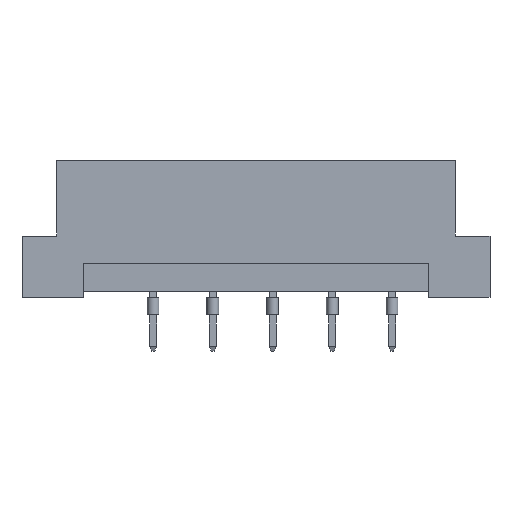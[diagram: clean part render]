
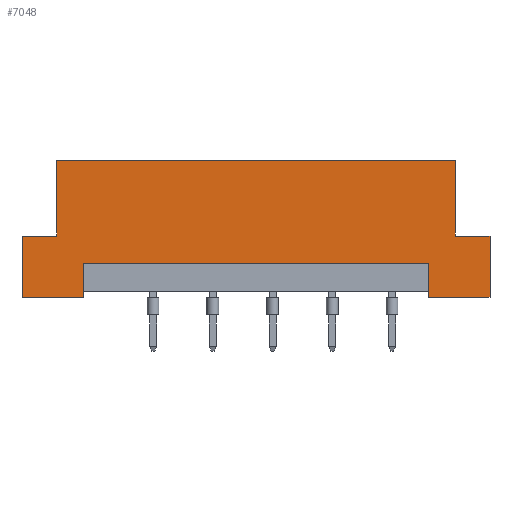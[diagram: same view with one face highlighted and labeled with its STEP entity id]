
A CAD part, front view. The second image highlights one B-rep face of the part: STEP entity #7048.
In plain terms, the highlighted planar face has unit normal (0, -1, 0).
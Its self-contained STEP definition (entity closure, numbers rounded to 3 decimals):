
#90 = DIRECTION ( 'NONE',  ( 0., 1., 0. ) ) ;
#134 = VERTEX_POINT ( 'NONE', #6791 ) ;
#160 = EDGE_CURVE ( 'NONE', #5860, #134, #2543, .T. ) ;
#199 = ORIENTED_EDGE ( 'NONE', *, *, #4637, .F. ) ;
#377 = VECTOR ( 'NONE', #6866, 1000. ) ;
#408 = LINE ( 'NONE', #2634, #3359 ) ;
#445 = ORIENTED_EDGE ( 'NONE', *, *, #2187, .F. ) ;
#552 = DIRECTION ( 'NONE',  ( -1., 0., 0. ) ) ;
#680 = VECTOR ( 'NONE', #4980, 1000. ) ;
#683 = ORIENTED_EDGE ( 'NONE', *, *, #3995, .F. ) ;
#708 = ORIENTED_EDGE ( 'NONE', *, *, #6460, .F. ) ;
#858 = VECTOR ( 'NONE', #6327, 1000. ) ;
#861 = VERTEX_POINT ( 'NONE', #6734 ) ;
#906 = CARTESIAN_POINT ( 'NONE',  ( 19.9, 0., 0. ) ) ;
#952 = LINE ( 'NONE', #2684, #6837 ) ;
#1167 = VERTEX_POINT ( 'NONE', #5324 ) ;
#1282 = LINE ( 'NONE', #3361, #4020 ) ;
#1418 = ORIENTED_EDGE ( 'NONE', *, *, #2986, .F. ) ;
#1699 = CARTESIAN_POINT ( 'NONE',  ( -16.94, 0., 11.6 ) ) ;
#1793 = ORIENTED_EDGE ( 'NONE', *, *, #6043, .F. ) ;
#2003 = LINE ( 'NONE', #2671, #4045 ) ;
#2011 = EDGE_LOOP ( 'NONE', ( #5216, #4098, #4525, #445, #6843, #6294, #1793, #5150, #199, #1418, #708, #683 ) ) ;
#2084 = DIRECTION ( 'NONE',  ( 0., 0., -1. ) ) ;
#2187 = EDGE_CURVE ( 'NONE', #4415, #5860, #4401, .T. ) ;
#2193 = LINE ( 'NONE', #3847, #4277 ) ;
#2227 = CARTESIAN_POINT ( 'NONE',  ( -16.94, 0., 5.2 ) ) ;
#2368 = CARTESIAN_POINT ( 'NONE',  ( -14.69, 0., 0.5 ) ) ;
#2543 = LINE ( 'NONE', #3081, #377 ) ;
#2559 = VERTEX_POINT ( 'NONE', #1699 ) ;
#2571 = DIRECTION ( 'NONE',  ( 1., 0., 0. ) ) ;
#2602 = DIRECTION ( 'NONE',  ( 1., 0., 0. ) ) ;
#2634 = CARTESIAN_POINT ( 'NONE',  ( -19.9, 0., 11.6 ) ) ;
#2671 = CARTESIAN_POINT ( 'NONE',  ( 19.9, 0., 5.2 ) ) ;
#2684 = CARTESIAN_POINT ( 'NONE',  ( 14.69, 0., 0.5 ) ) ;
#2693 = CARTESIAN_POINT ( 'NONE',  ( -19.9, 0., 5.2 ) ) ;
#2758 = VERTEX_POINT ( 'NONE', #2227 ) ;
#2821 = VECTOR ( 'NONE', #6826, 1000. ) ;
#2983 = CARTESIAN_POINT ( 'NONE',  ( 16.94, 0., 5.2 ) ) ;
#2986 = EDGE_CURVE ( 'NONE', #4608, #861, #1282, .T. ) ;
#3016 = LINE ( 'NONE', #6293, #858 ) ;
#3081 = CARTESIAN_POINT ( 'NONE',  ( -19.9, 0., 0. ) ) ;
#3222 = CARTESIAN_POINT ( 'NONE',  ( 14.69, 0., 2.9 ) ) ;
#3250 = CARTESIAN_POINT ( 'NONE',  ( -14.69, 0., 2.9 ) ) ;
#3359 = VECTOR ( 'NONE', #2571, 1000. ) ;
#3361 = CARTESIAN_POINT ( 'NONE',  ( -19.9, 0., 0. ) ) ;
#3554 = VERTEX_POINT ( 'NONE', #2983 ) ;
#3674 = VERTEX_POINT ( 'NONE', #5849 ) ;
#3776 = EDGE_CURVE ( 'NONE', #5462, #134, #952, .T. ) ;
#3824 = VECTOR ( 'NONE', #7015, 1000. ) ;
#3847 = CARTESIAN_POINT ( 'NONE',  ( -19.9, 0., 0. ) ) ;
#3926 = VECTOR ( 'NONE', #552, 1000. ) ;
#3995 = EDGE_CURVE ( 'NONE', #5937, #3674, #5525, .T. ) ;
#4020 = VECTOR ( 'NONE', #6732, 1000. ) ;
#4045 = VECTOR ( 'NONE', #2602, 1000. ) ;
#4063 = CARTESIAN_POINT ( 'NONE',  ( 16.94, 0., 5.2 ) ) ;
#4098 = ORIENTED_EDGE ( 'NONE', *, *, #3776, .T. ) ;
#4133 = EDGE_CURVE ( 'NONE', #3554, #1167, #5167, .T. ) ;
#4272 = CARTESIAN_POINT ( 'NONE',  ( 14.69, 0., 2.9 ) ) ;
#4277 = VECTOR ( 'NONE', #6026, 1000. ) ;
#4401 = LINE ( 'NONE', #6594, #680 ) ;
#4415 = VERTEX_POINT ( 'NONE', #4912 ) ;
#4480 = FACE_OUTER_BOUND ( 'NONE', #2011, .T. ) ;
#4525 = ORIENTED_EDGE ( 'NONE', *, *, #160, .F. ) ;
#4545 = PLANE ( 'NONE',  #5776 ) ;
#4608 = VERTEX_POINT ( 'NONE', #4969 ) ;
#4637 = EDGE_CURVE ( 'NONE', #861, #2758, #6543, .T. ) ;
#4912 = CARTESIAN_POINT ( 'NONE',  ( 19.9, 0., 5.2 ) ) ;
#4969 = CARTESIAN_POINT ( 'NONE',  ( -19.9, 0., 0. ) ) ;
#4980 = DIRECTION ( 'NONE',  ( 0., 0., -1. ) ) ;
#5150 = ORIENTED_EDGE ( 'NONE', *, *, #6751, .F. ) ;
#5167 = LINE ( 'NONE', #4063, #6716 ) ;
#5216 = ORIENTED_EDGE ( 'NONE', *, *, #5534, .F. ) ;
#5324 = CARTESIAN_POINT ( 'NONE',  ( 16.94, 0., 11.6 ) ) ;
#5445 = LINE ( 'NONE', #4272, #3926 ) ;
#5462 = VERTEX_POINT ( 'NONE', #3222 ) ;
#5525 = LINE ( 'NONE', #2368, #2821 ) ;
#5534 = EDGE_CURVE ( 'NONE', #5462, #5937, #5445, .T. ) ;
#5776 = AXIS2_PLACEMENT_3D ( 'NONE', #6058, #90, #6748 ) ;
#5849 = CARTESIAN_POINT ( 'NONE',  ( -14.69, 0., 0. ) ) ;
#5860 = VERTEX_POINT ( 'NONE', #906 ) ;
#5937 = VERTEX_POINT ( 'NONE', #3250 ) ;
#6025 = EDGE_CURVE ( 'NONE', #3554, #4415, #2003, .T. ) ;
#6026 = DIRECTION ( 'NONE',  ( -1., 0., 0. ) ) ;
#6043 = EDGE_CURVE ( 'NONE', #2559, #1167, #408, .T. ) ;
#6058 = CARTESIAN_POINT ( 'NONE',  ( -19.9, 0., 11.6 ) ) ;
#6247 = DIRECTION ( 'NONE',  ( 0., 0., 1. ) ) ;
#6293 = CARTESIAN_POINT ( 'NONE',  ( -16.94, 0., 5.2 ) ) ;
#6294 = ORIENTED_EDGE ( 'NONE', *, *, #4133, .T. ) ;
#6327 = DIRECTION ( 'NONE',  ( 0., 0., 1. ) ) ;
#6460 = EDGE_CURVE ( 'NONE', #3674, #4608, #2193, .T. ) ;
#6543 = LINE ( 'NONE', #2693, #3824 ) ;
#6594 = CARTESIAN_POINT ( 'NONE',  ( 19.9, 0., 0. ) ) ;
#6716 = VECTOR ( 'NONE', #6247, 1000. ) ;
#6732 = DIRECTION ( 'NONE',  ( 0., 0., 1. ) ) ;
#6734 = CARTESIAN_POINT ( 'NONE',  ( -19.9, 0., 5.2 ) ) ;
#6748 = DIRECTION ( 'NONE',  ( 0., 0., 1. ) ) ;
#6751 = EDGE_CURVE ( 'NONE', #2758, #2559, #3016, .T. ) ;
#6791 = CARTESIAN_POINT ( 'NONE',  ( 14.69, 0., 0. ) ) ;
#6826 = DIRECTION ( 'NONE',  ( 0., 0., -1. ) ) ;
#6837 = VECTOR ( 'NONE', #2084, 1000. ) ;
#6843 = ORIENTED_EDGE ( 'NONE', *, *, #6025, .F. ) ;
#6866 = DIRECTION ( 'NONE',  ( -1., 0., 0. ) ) ;
#7015 = DIRECTION ( 'NONE',  ( 1., 0., 0. ) ) ;
#7048 = ADVANCED_FACE ( 'NONE', ( #4480 ), #4545, .F. ) ;
